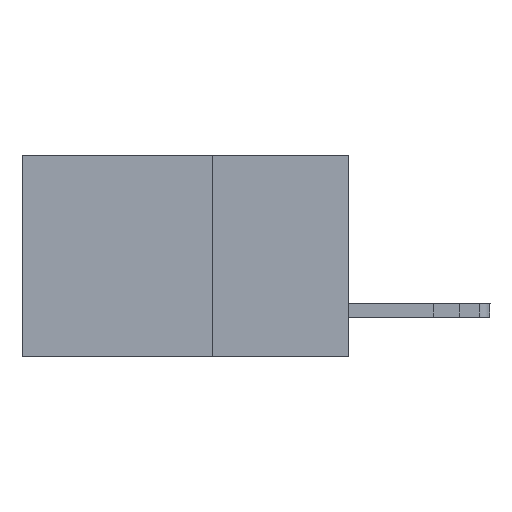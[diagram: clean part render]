
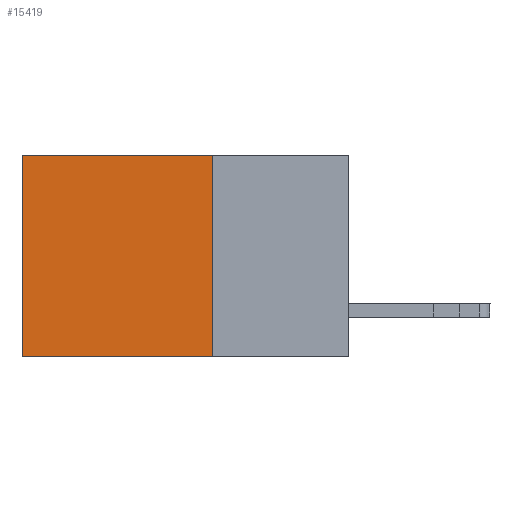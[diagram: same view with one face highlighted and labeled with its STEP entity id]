
A CAD part, left-side view. The second image highlights one B-rep face of the part: STEP entity #15419.
In plain terms, the highlighted planar face has unit normal (-1, 0, 0).
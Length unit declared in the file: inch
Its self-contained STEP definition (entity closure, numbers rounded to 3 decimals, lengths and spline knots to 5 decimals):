
#699 = VERTEX_POINT ( 'NONE', #14210 ) ;
#1069 = LINE ( 'NONE', #6308, #4427 ) ;
#2004 = LINE ( 'NONE', #8329, #5322 ) ;
#2881 = AXIS2_PLACEMENT_3D ( 'NONE', #4129, #14076, #5576 ) ;
#3332 = EDGE_CURVE ( 'NONE', #18162, #9847, #2004, .T. ) ;
#4075 = PLANE ( 'NONE',  #2881 ) ;
#4129 = CARTESIAN_POINT ( 'NONE',  ( 0.2615, 0.25, -0.37 ) ) ;
#4427 = VECTOR ( 'NONE', #6259, 39.37008 ) ;
#4711 = EDGE_LOOP ( 'NONE', ( #10421, #4732, #11437, #14137 ) ) ;
#4732 = ORIENTED_EDGE ( 'NONE', *, *, #8396, .F. ) ;
#4922 = CARTESIAN_POINT ( 'NONE',  ( 0.2615, 0.6, -0.37 ) ) ;
#5322 = VECTOR ( 'NONE', #8306, 39.37008 ) ;
#5576 = DIRECTION ( 'NONE',  ( 0., 0., -1. ) ) ;
#6259 = DIRECTION ( 'NONE',  ( 0., 1., 0. ) ) ;
#6308 = CARTESIAN_POINT ( 'NONE',  ( 0.2615, 0.25, -0.37 ) ) ;
#7168 = LINE ( 'NONE', #12123, #10956 ) ;
#8239 = FACE_OUTER_BOUND ( 'NONE', #4711, .T. ) ;
#8306 = DIRECTION ( 'NONE',  ( 0., 1., 0. ) ) ;
#8329 = CARTESIAN_POINT ( 'NONE',  ( 0.2615, 0.25, 0. ) ) ;
#8396 = EDGE_CURVE ( 'NONE', #17721, #699, #1069, .T. ) ;
#8679 = CARTESIAN_POINT ( 'NONE',  ( 0.2615, 0.6, 0. ) ) ;
#9211 = CARTESIAN_POINT ( 'NONE',  ( 0.2615, 0.25, 0. ) ) ;
#9674 = CARTESIAN_POINT ( 'NONE',  ( 0.2615, 0.25, -0.37 ) ) ;
#9847 = VERTEX_POINT ( 'NONE', #8679 ) ;
#10421 = ORIENTED_EDGE ( 'NONE', *, *, #13018, .T. ) ;
#10956 = VECTOR ( 'NONE', #16359, 39.37008 ) ;
#11437 = ORIENTED_EDGE ( 'NONE', *, *, #12414, .F. ) ;
#12123 = CARTESIAN_POINT ( 'NONE',  ( 0.2615, 0.25, -0.37 ) ) ;
#12414 = EDGE_CURVE ( 'NONE', #18162, #17721, #7168, .T. ) ;
#13018 = EDGE_CURVE ( 'NONE', #9847, #699, #17990, .T. ) ;
#14076 = DIRECTION ( 'NONE',  ( 1., 0., 0. ) ) ;
#14137 = ORIENTED_EDGE ( 'NONE', *, *, #3332, .T. ) ;
#14210 = CARTESIAN_POINT ( 'NONE',  ( 0.2615, 0.6, -0.37 ) ) ;
#14262 = VECTOR ( 'NONE', #16279, 39.37008 ) ;
#15419 = ADVANCED_FACE ( 'NONE', ( #8239 ), #4075, .F. ) ;
#16279 = DIRECTION ( 'NONE',  ( 0., 0., -1. ) ) ;
#16359 = DIRECTION ( 'NONE',  ( 0., 0., -1. ) ) ;
#17721 = VERTEX_POINT ( 'NONE', #9674 ) ;
#17990 = LINE ( 'NONE', #4922, #14262 ) ;
#18162 = VERTEX_POINT ( 'NONE', #9211 ) ;
